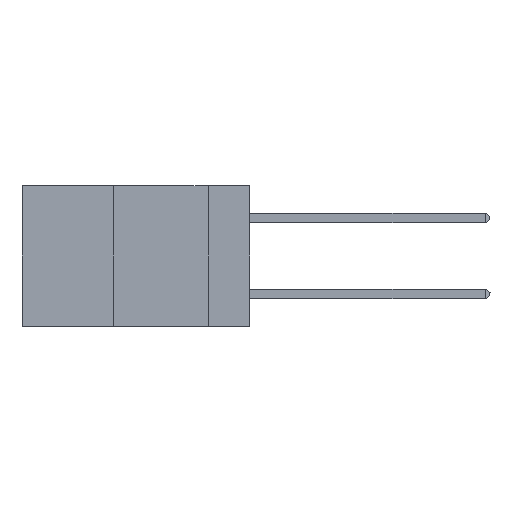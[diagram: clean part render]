
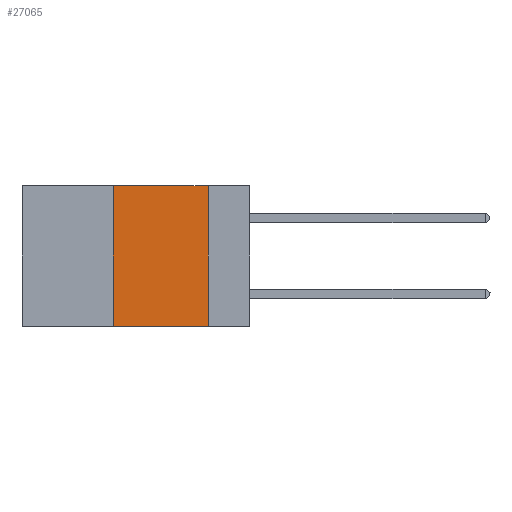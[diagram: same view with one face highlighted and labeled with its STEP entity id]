
A CAD part, left-side view. The second image highlights one B-rep face of the part: STEP entity #27065.
In plain terms, the highlighted planar face has unit normal (-1, 0, 0).
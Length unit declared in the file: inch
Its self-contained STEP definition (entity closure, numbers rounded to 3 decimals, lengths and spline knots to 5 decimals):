
#787 = CARTESIAN_POINT ( 'NONE',  ( 0., 0.11, 0. ) ) ;
#1724 = EDGE_CURVE ( 'NONE', #7542, #4404, #15310, .T. ) ;
#2484 = FACE_OUTER_BOUND ( 'NONE', #18125, .T. ) ;
#2924 = CARTESIAN_POINT ( 'NONE',  ( 0., 0.6, -0.37 ) ) ;
#3460 = CARTESIAN_POINT ( 'NONE',  ( 0., 0.36, -0.37 ) ) ;
#3907 = ORIENTED_EDGE ( 'NONE', *, *, #1724, .F. ) ;
#4041 = VECTOR ( 'NONE', #21854, 39.37008 ) ;
#4331 = DIRECTION ( 'NONE',  ( 0., 0., 1. ) ) ;
#4404 = VERTEX_POINT ( 'NONE', #787 ) ;
#4442 = ORIENTED_EDGE ( 'NONE', *, *, #6926, .F. ) ;
#4860 = DIRECTION ( 'NONE',  ( 0., -1., 0. ) ) ;
#5068 = DIRECTION ( 'NONE',  ( 0., -1., 0. ) ) ;
#6538 = PLANE ( 'NONE',  #11314 ) ;
#6926 = EDGE_CURVE ( 'NONE', #4404, #15307, #15865, .T. ) ;
#7542 = VERTEX_POINT ( 'NONE', #12494 ) ;
#8648 = DIRECTION ( 'NONE',  ( 1., 0., 0. ) ) ;
#10796 = LINE ( 'NONE', #2924, #21253 ) ;
#11314 = AXIS2_PLACEMENT_3D ( 'NONE', #21168, #8648, #23288 ) ;
#12494 = CARTESIAN_POINT ( 'NONE',  ( 0., 0.36, 0. ) ) ;
#12818 = ORIENTED_EDGE ( 'NONE', *, *, #14973, .F. ) ;
#14788 = CARTESIAN_POINT ( 'NONE',  ( 0., 0.36, 0. ) ) ;
#14973 = EDGE_CURVE ( 'NONE', #16374, #7542, #21503, .T. ) ;
#15306 = CARTESIAN_POINT ( 'NONE',  ( 0., 0.6, 0. ) ) ;
#15307 = VERTEX_POINT ( 'NONE', #20078 ) ;
#15310 = LINE ( 'NONE', #15306, #16616 ) ;
#15865 = LINE ( 'NONE', #19749, #4041 ) ;
#16374 = VERTEX_POINT ( 'NONE', #3460 ) ;
#16616 = VECTOR ( 'NONE', #4860, 39.37008 ) ;
#17416 = EDGE_CURVE ( 'NONE', #16374, #15307, #10796, .T. ) ;
#18125 = EDGE_LOOP ( 'NONE', ( #4442, #3907, #12818, #20981 ) ) ;
#19749 = CARTESIAN_POINT ( 'NONE',  ( 0., 0.11, 0. ) ) ;
#20078 = CARTESIAN_POINT ( 'NONE',  ( 0., 0.11, -0.37 ) ) ;
#20981 = ORIENTED_EDGE ( 'NONE', *, *, #17416, .T. ) ;
#21168 = CARTESIAN_POINT ( 'NONE',  ( 0., 0.6, 0. ) ) ;
#21253 = VECTOR ( 'NONE', #5068, 39.37008 ) ;
#21503 = LINE ( 'NONE', #14788, #26402 ) ;
#21854 = DIRECTION ( 'NONE',  ( 0., 0., -1. ) ) ;
#23288 = DIRECTION ( 'NONE',  ( 0., 0., -1. ) ) ;
#26402 = VECTOR ( 'NONE', #4331, 39.37008 ) ;
#27065 = ADVANCED_FACE ( 'NONE', ( #2484 ), #6538, .F. ) ;
